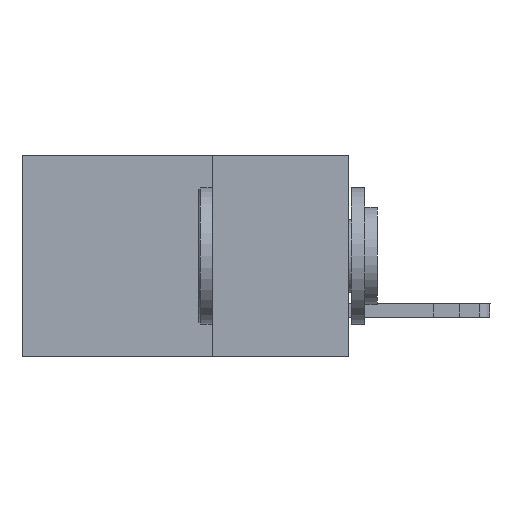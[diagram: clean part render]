
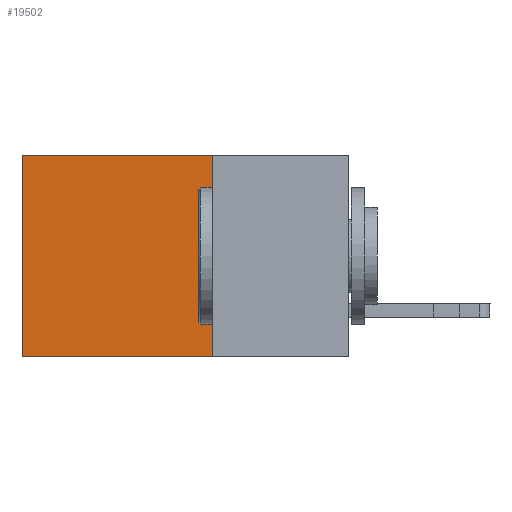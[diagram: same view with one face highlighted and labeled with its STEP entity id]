
A CAD part, left-side view. The second image highlights one B-rep face of the part: STEP entity #19502.
In plain terms, the highlighted planar face has unit normal (-1, 0, 0).
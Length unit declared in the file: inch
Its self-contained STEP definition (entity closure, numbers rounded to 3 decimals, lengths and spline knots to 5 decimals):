
#438 = EDGE_CURVE ( 'NONE', #12703, #20920, #4555, .T. ) ;
#1221 = VECTOR ( 'NONE', #23399, 39.37008 ) ;
#1668 = VECTOR ( 'NONE', #19476, 39.37008 ) ;
#1866 = EDGE_CURVE ( 'NONE', #20920, #15261, #6559, .T. ) ;
#2237 = DIRECTION ( 'NONE',  ( 1., 0., 0. ) ) ;
#2680 = CARTESIAN_POINT ( 'NONE',  ( 0.298, 0.6, 0. ) ) ;
#2962 = CARTESIAN_POINT ( 'NONE',  ( 0.298, 0.6, 0. ) ) ;
#3205 = CARTESIAN_POINT ( 'NONE',  ( 0.298, 0.25, -0.37 ) ) ;
#4555 = LINE ( 'NONE', #11145, #23555 ) ;
#5042 = ORIENTED_EDGE ( 'NONE', *, *, #19904, .T. ) ;
#5553 = DIRECTION ( 'NONE',  ( 0., 0., -1. ) ) ;
#5764 = CARTESIAN_POINT ( 'NONE',  ( 0.298, 0.25, -0.37 ) ) ;
#6424 = EDGE_CURVE ( 'NONE', #15894, #15261, #16791, .T. ) ;
#6559 = LINE ( 'NONE', #3205, #1668 ) ;
#7387 = FACE_OUTER_BOUND ( 'NONE', #16958, .T. ) ;
#7670 = LINE ( 'NONE', #17933, #15439 ) ;
#8657 = ORIENTED_EDGE ( 'NONE', *, *, #1866, .F. ) ;
#9107 = AXIS2_PLACEMENT_3D ( 'NONE', #11207, #2237, #5553 ) ;
#11145 = CARTESIAN_POINT ( 'NONE',  ( 0.298, 0.25, 0. ) ) ;
#11207 = CARTESIAN_POINT ( 'NONE',  ( 0.298, 0.25, 0. ) ) ;
#11863 = CARTESIAN_POINT ( 'NONE',  ( 0.298, 0.25, 0. ) ) ;
#12703 = VERTEX_POINT ( 'NONE', #11863 ) ;
#13203 = CARTESIAN_POINT ( 'NONE',  ( 0.298, 0.6, -0.37 ) ) ;
#13271 = PLANE ( 'NONE',  #9107 ) ;
#14757 = ORIENTED_EDGE ( 'NONE', *, *, #6424, .T. ) ;
#15261 = VERTEX_POINT ( 'NONE', #13203 ) ;
#15439 = VECTOR ( 'NONE', #21655, 39.37008 ) ;
#15894 = VERTEX_POINT ( 'NONE', #2680 ) ;
#16791 = LINE ( 'NONE', #2962, #1221 ) ;
#16958 = EDGE_LOOP ( 'NONE', ( #14757, #8657, #23341, #5042 ) ) ;
#17933 = CARTESIAN_POINT ( 'NONE',  ( 0.298, 0.25, 0. ) ) ;
#19476 = DIRECTION ( 'NONE',  ( 0., 1., 0. ) ) ;
#19502 = ADVANCED_FACE ( 'NONE', ( #7387 ), #13271, .F. ) ;
#19904 = EDGE_CURVE ( 'NONE', #12703, #15894, #7670, .T. ) ;
#20920 = VERTEX_POINT ( 'NONE', #5764 ) ;
#21655 = DIRECTION ( 'NONE',  ( 0., 1., 0. ) ) ;
#22316 = DIRECTION ( 'NONE',  ( 0., 0., -1. ) ) ;
#23341 = ORIENTED_EDGE ( 'NONE', *, *, #438, .F. ) ;
#23399 = DIRECTION ( 'NONE',  ( 0., 0., -1. ) ) ;
#23555 = VECTOR ( 'NONE', #22316, 39.37008 ) ;
